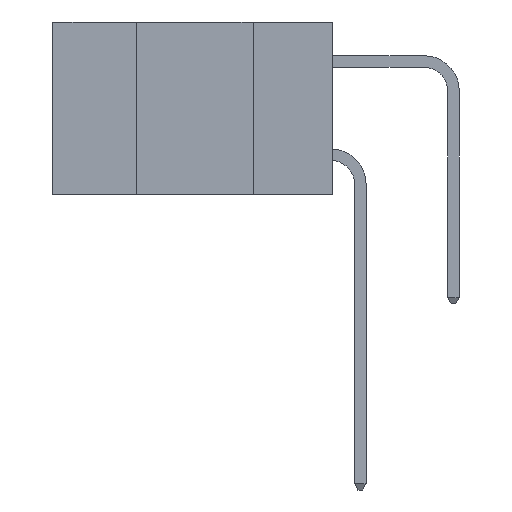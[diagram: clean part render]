
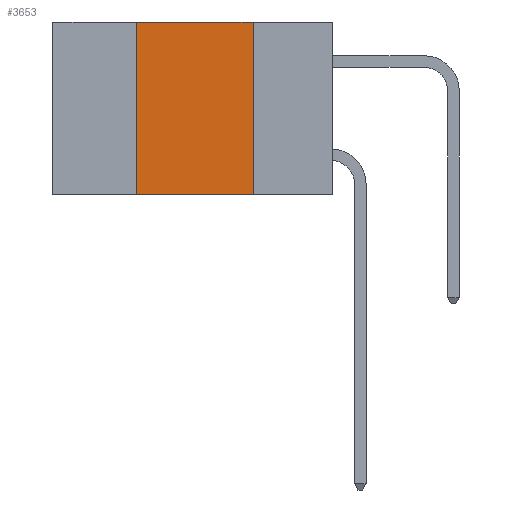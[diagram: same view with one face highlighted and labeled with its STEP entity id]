
A CAD part, left-side view. The second image highlights one B-rep face of the part: STEP entity #3653.
In plain terms, the highlighted planar face has unit normal (-1, 0, 0).
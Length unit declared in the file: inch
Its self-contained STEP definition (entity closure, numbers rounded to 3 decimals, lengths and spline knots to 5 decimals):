
#190 = EDGE_LOOP ( 'NONE', ( #15235, #15564, #3109, #549 ) ) ;
#255 = VERTEX_POINT ( 'NONE', #13428 ) ;
#424 = EDGE_CURVE ( 'NONE', #7410, #10550, #5494, .T. ) ;
#549 = ORIENTED_EDGE ( 'NONE', *, *, #11737, .T. ) ;
#872 = VERTEX_POINT ( 'NONE', #10385 ) ;
#945 = EDGE_CURVE ( 'NONE', #255, #7410, #13310, .T. ) ;
#1260 = EDGE_CURVE ( 'NONE', #10550, #872, #9470, .T. ) ;
#3109 = ORIENTED_EDGE ( 'NONE', *, *, #945, .F. ) ;
#3653 = ADVANCED_FACE ( 'NONE', ( #15205 ), #10188, .F. ) ;
#4940 = CARTESIAN_POINT ( 'NONE',  ( 0., 0.42, 0. ) ) ;
#5494 = LINE ( 'NONE', #13156, #7950 ) ;
#5854 = VECTOR ( 'NONE', #9693, 39.37008 ) ;
#6800 = VECTOR ( 'NONE', #10826, 39.37008 ) ;
#7410 = VERTEX_POINT ( 'NONE', #4940 ) ;
#7950 = VECTOR ( 'NONE', #14455, 39.37008 ) ;
#7954 = DIRECTION ( 'NONE',  ( 0., -1., 0. ) ) ;
#9470 = LINE ( 'NONE', #9752, #5854 ) ;
#9693 = DIRECTION ( 'NONE',  ( 0., 0., -1. ) ) ;
#9752 = CARTESIAN_POINT ( 'NONE',  ( 0., 0.17, -0.37 ) ) ;
#9987 = DIRECTION ( 'NONE',  ( 0., 0., -1. ) ) ;
#10039 = DIRECTION ( 'NONE',  ( 1., 0., 0. ) ) ;
#10135 = CARTESIAN_POINT ( 'NONE',  ( 0., 0.6, 0. ) ) ;
#10188 = PLANE ( 'NONE',  #13264 ) ;
#10385 = CARTESIAN_POINT ( 'NONE',  ( 0., 0.17, -0.37 ) ) ;
#10550 = VERTEX_POINT ( 'NONE', #13056 ) ;
#10826 = DIRECTION ( 'NONE',  ( 0., 0., 1. ) ) ;
#11034 = LINE ( 'NONE', #15155, #14260 ) ;
#11737 = EDGE_CURVE ( 'NONE', #255, #872, #11034, .T. ) ;
#11839 = CARTESIAN_POINT ( 'NONE',  ( 0., 0.42, -0.37 ) ) ;
#13056 = CARTESIAN_POINT ( 'NONE',  ( 0., 0.17, 0. ) ) ;
#13156 = CARTESIAN_POINT ( 'NONE',  ( 0., 0.6, 0. ) ) ;
#13264 = AXIS2_PLACEMENT_3D ( 'NONE', #10135, #10039, #9987 ) ;
#13310 = LINE ( 'NONE', #11839, #6800 ) ;
#13428 = CARTESIAN_POINT ( 'NONE',  ( 0., 0.42, -0.37 ) ) ;
#14260 = VECTOR ( 'NONE', #7954, 39.37008 ) ;
#14455 = DIRECTION ( 'NONE',  ( 0., -1., 0. ) ) ;
#15155 = CARTESIAN_POINT ( 'NONE',  ( 0., 0.6, -0.37 ) ) ;
#15205 = FACE_OUTER_BOUND ( 'NONE', #190, .T. ) ;
#15235 = ORIENTED_EDGE ( 'NONE', *, *, #1260, .F. ) ;
#15564 = ORIENTED_EDGE ( 'NONE', *, *, #424, .F. ) ;
